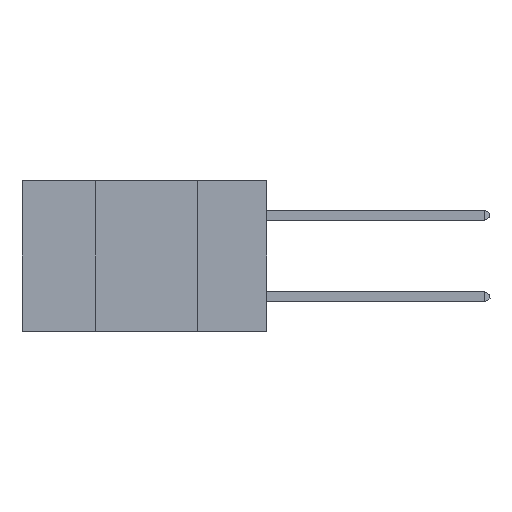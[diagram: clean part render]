
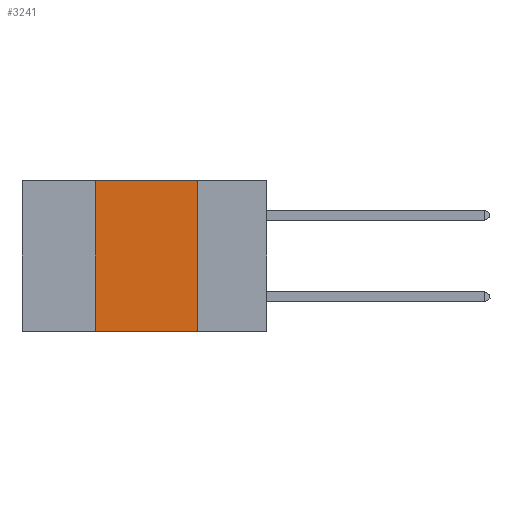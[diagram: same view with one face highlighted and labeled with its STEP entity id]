
A CAD part, left-side view. The second image highlights one B-rep face of the part: STEP entity #3241.
In plain terms, the highlighted planar face has unit normal (-1, 0, 0).
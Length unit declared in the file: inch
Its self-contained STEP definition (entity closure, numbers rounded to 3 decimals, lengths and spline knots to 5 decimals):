
#702 = VERTEX_POINT ( 'NONE', #5001 ) ;
#912 = VECTOR ( 'NONE', #2213, 39.37008 ) ;
#1013 = DIRECTION ( 'NONE',  ( 0., 0., -1. ) ) ;
#1146 = ORIENTED_EDGE ( 'NONE', *, *, #15397, .T. ) ;
#1701 = LINE ( 'NONE', #3650, #11488 ) ;
#1991 = LINE ( 'NONE', #11707, #13432 ) ;
#2213 = DIRECTION ( 'NONE',  ( 0., -1., 0. ) ) ;
#2777 = VERTEX_POINT ( 'NONE', #12252 ) ;
#3241 = ADVANCED_FACE ( 'NONE', ( #15174 ), #6076, .F. ) ;
#3650 = CARTESIAN_POINT ( 'NONE',  ( 0., 0.6, 0. ) ) ;
#4418 = CARTESIAN_POINT ( 'NONE',  ( 0., 0.42, 0. ) ) ;
#4691 = DIRECTION ( 'NONE',  ( 0., -1., 0. ) ) ;
#5001 = CARTESIAN_POINT ( 'NONE',  ( 0., 0.42, -0.37 ) ) ;
#5782 = DIRECTION ( 'NONE',  ( 0., 0., -1. ) ) ;
#5890 = DIRECTION ( 'NONE',  ( 1., 0., 0. ) ) ;
#5902 = CARTESIAN_POINT ( 'NONE',  ( 0., 0.42, 0. ) ) ;
#6076 = PLANE ( 'NONE',  #6352 ) ;
#6267 = CARTESIAN_POINT ( 'NONE',  ( 0., 0.17, 0. ) ) ;
#6352 = AXIS2_PLACEMENT_3D ( 'NONE', #8468, #5890, #1013 ) ;
#6638 = LINE ( 'NONE', #12960, #912 ) ;
#7043 = ORIENTED_EDGE ( 'NONE', *, *, #7911, .F. ) ;
#7911 = EDGE_CURVE ( 'NONE', #14884, #13319, #1701, .T. ) ;
#7916 = VECTOR ( 'NONE', #13797, 39.37008 ) ;
#8468 = CARTESIAN_POINT ( 'NONE',  ( 0., 0.6, 0. ) ) ;
#8851 = LINE ( 'NONE', #4418, #7916 ) ;
#9032 = ORIENTED_EDGE ( 'NONE', *, *, #11803, .F. ) ;
#10357 = ORIENTED_EDGE ( 'NONE', *, *, #15364, .F. ) ;
#11488 = VECTOR ( 'NONE', #4691, 39.37008 ) ;
#11707 = CARTESIAN_POINT ( 'NONE',  ( 0., 0.17, 0. ) ) ;
#11803 = EDGE_CURVE ( 'NONE', #13319, #2777, #1991, .T. ) ;
#12252 = CARTESIAN_POINT ( 'NONE',  ( 0., 0.17, -0.37 ) ) ;
#12960 = CARTESIAN_POINT ( 'NONE',  ( 0., 0.6, -0.37 ) ) ;
#13319 = VERTEX_POINT ( 'NONE', #6267 ) ;
#13432 = VECTOR ( 'NONE', #5782, 39.37008 ) ;
#13797 = DIRECTION ( 'NONE',  ( 0., 0., 1. ) ) ;
#14884 = VERTEX_POINT ( 'NONE', #5902 ) ;
#14952 = EDGE_LOOP ( 'NONE', ( #9032, #7043, #10357, #1146 ) ) ;
#15174 = FACE_OUTER_BOUND ( 'NONE', #14952, .T. ) ;
#15364 = EDGE_CURVE ( 'NONE', #702, #14884, #8851, .T. ) ;
#15397 = EDGE_CURVE ( 'NONE', #702, #2777, #6638, .T. ) ;
